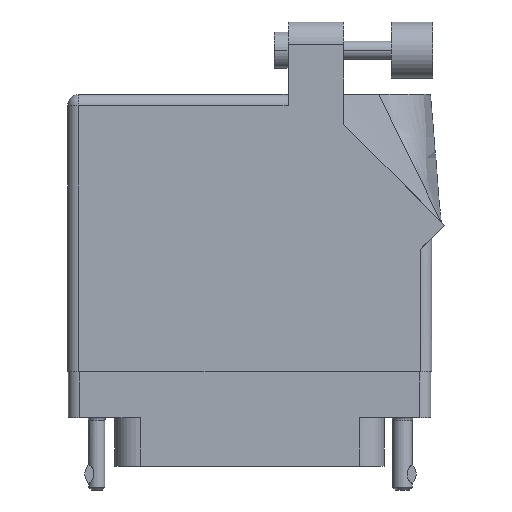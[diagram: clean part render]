
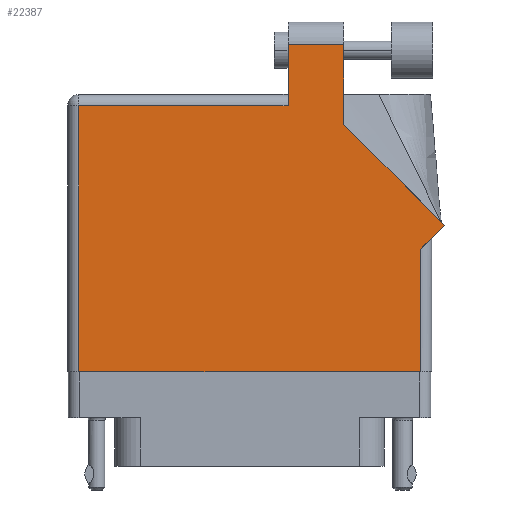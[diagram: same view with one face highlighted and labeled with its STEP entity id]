
A CAD part, front view. The second image highlights one B-rep face of the part: STEP entity #22387.
In plain terms, the highlighted face is planar.
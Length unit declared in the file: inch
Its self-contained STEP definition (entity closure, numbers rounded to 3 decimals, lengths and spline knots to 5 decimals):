
#265 = EDGE_CURVE ( 'NONE', #39136, #20996, #43866, .T. ) ;
#532 = EDGE_CURVE ( 'NONE', #18639, #32042, #30195, .T. ) ;
#1149 = CARTESIAN_POINT ( 'NONE',  ( 0.943, -0.1, 0.455 ) ) ;
#1171 = LINE ( 'NONE', #38625, #28031 ) ;
#1487 = DIRECTION ( 'NONE',  ( 1., 0., 0. ) ) ;
#1673 = CARTESIAN_POINT ( 'NONE',  ( -0.943, -0.1, 0.455 ) ) ;
#2623 = CARTESIAN_POINT ( 'NONE',  ( 0.212, 1.368, 0.455 ) ) ;
#3544 = ORIENTED_EDGE ( 'NONE', *, *, #8520, .T. ) ;
#4183 = ORIENTED_EDGE ( 'NONE', *, *, #13772, .T. ) ;
#4463 = VERTEX_POINT ( 'NONE', #1673 ) ;
#5615 = VECTOR ( 'NONE', #8112, 39.37008 ) ;
#5845 = PLANE ( 'NONE',  #21014 ) ;
#7066 = CARTESIAN_POINT ( 'NONE',  ( 0.943, 0.575, 0.455 ) ) ;
#7652 = VERTEX_POINT ( 'NONE', #2623 ) ;
#7883 = DIRECTION ( 'NONE',  ( -1., 0., 0. ) ) ;
#8112 = DIRECTION ( 'NONE',  ( 0.707, 0.707, 0. ) ) ;
#8467 = EDGE_CURVE ( 'NONE', #43253, #4463, #43627, .T. ) ;
#8520 = EDGE_CURVE ( 'NONE', #4463, #28490, #17906, .T. ) ;
#8932 = ORIENTED_EDGE ( 'NONE', *, *, #25305, .T. ) ;
#8941 = VECTOR ( 'NONE', #26230, 39.37008 ) ;
#9267 = CARTESIAN_POINT ( 'NONE',  ( 0.212, 1.705, 0.455 ) ) ;
#9564 = ORIENTED_EDGE ( 'NONE', *, *, #265, .T. ) ;
#10597 = LINE ( 'NONE', #32821, #8941 ) ;
#10769 = VECTOR ( 'NONE', #27896, 39.37008 ) ;
#13772 = EDGE_CURVE ( 'NONE', #20996, #18639, #31195, .T. ) ;
#14037 = CARTESIAN_POINT ( 'NONE',  ( 0.519, 1.26442, 0.455 ) ) ;
#15099 = CARTESIAN_POINT ( 'NONE',  ( -0.943, -0.1, 0.455 ) ) ;
#16652 = DIRECTION ( 'NONE',  ( -1., 0., 0. ) ) ;
#17893 = LINE ( 'NONE', #20901, #10769 ) ;
#17906 = LINE ( 'NONE', #26004, #32177 ) ;
#18501 = DIRECTION ( 'NONE',  ( 0., -1., 0. ) ) ;
#18639 = VERTEX_POINT ( 'NONE', #24933 ) ;
#20701 = VECTOR ( 'NONE', #18501, 39.37008 ) ;
#20901 = CARTESIAN_POINT ( 'NONE',  ( 0.943, 0.637, 0.455 ) ) ;
#20996 = VERTEX_POINT ( 'NONE', #33366 ) ;
#21014 = AXIS2_PLACEMENT_3D ( 'NONE', #30618, #40550, #16652 ) ;
#21344 = ORIENTED_EDGE ( 'NONE', *, *, #8467, .T. ) ;
#22387 = ADVANCED_FACE ( 'NONE', ( #24769 ), #5845, .F. ) ;
#23096 = CARTESIAN_POINT ( 'NONE',  ( 1.07571, 0.70771, 0.455 ) ) ;
#23632 = VECTOR ( 'NONE', #40493, 39.37008 ) ;
#24769 = FACE_OUTER_BOUND ( 'NONE', #45059, .T. ) ;
#24906 = EDGE_CURVE ( 'NONE', #40046, #39136, #28618, .T. ) ;
#24933 = CARTESIAN_POINT ( 'NONE',  ( 0.519, 1.705, 0.455 ) ) ;
#25305 = EDGE_CURVE ( 'NONE', #7652, #43253, #1171, .T. ) ;
#25799 = VECTOR ( 'NONE', #44161, 39.37008 ) ;
#26004 = CARTESIAN_POINT ( 'NONE',  ( -1.005, -0.1, 0.455 ) ) ;
#26230 = DIRECTION ( 'NONE',  ( 0., -1., 0. ) ) ;
#27896 = DIRECTION ( 'NONE',  ( 0., 1., 0. ) ) ;
#28031 = VECTOR ( 'NONE', #7883, 39.37008 ) ;
#28490 = VERTEX_POINT ( 'NONE', #1149 ) ;
#28618 = LINE ( 'NONE', #35818, #5615 ) ;
#30195 = LINE ( 'NONE', #9267, #25799 ) ;
#30618 = CARTESIAN_POINT ( 'NONE',  ( -1.005, 1.43, 0.455 ) ) ;
#31195 = LINE ( 'NONE', #14037, #33373 ) ;
#31526 = DIRECTION ( 'NONE',  ( 0., 1., 0. ) ) ;
#32042 = VERTEX_POINT ( 'NONE', #44549 ) ;
#32177 = VECTOR ( 'NONE', #1487, 39.37008 ) ;
#32821 = CARTESIAN_POINT ( 'NONE',  ( 0.212, 1.43, 0.455 ) ) ;
#33366 = CARTESIAN_POINT ( 'NONE',  ( 0.519, 1.26442, 0.455 ) ) ;
#33373 = VECTOR ( 'NONE', #31526, 39.37008 ) ;
#33457 = ORIENTED_EDGE ( 'NONE', *, *, #532, .T. ) ;
#35353 = EDGE_CURVE ( 'NONE', #28490, #40046, #17893, .T. ) ;
#35818 = CARTESIAN_POINT ( 'NONE',  ( 1.005, 0.637, 0.455 ) ) ;
#36095 = ORIENTED_EDGE ( 'NONE', *, *, #37046, .T. ) ;
#36755 = ORIENTED_EDGE ( 'NONE', *, *, #35353, .T. ) ;
#37046 = EDGE_CURVE ( 'NONE', #32042, #7652, #10597, .T. ) ;
#38625 = CARTESIAN_POINT ( 'NONE',  ( -1.005, 1.368, 0.455 ) ) ;
#39136 = VERTEX_POINT ( 'NONE', #42745 ) ;
#40046 = VERTEX_POINT ( 'NONE', #7066 ) ;
#40493 = DIRECTION ( 'NONE',  ( -0.707, 0.707, 0. ) ) ;
#40550 = DIRECTION ( 'NONE',  ( 0., 0., -1. ) ) ;
#40602 = CARTESIAN_POINT ( 'NONE',  ( -0.943, 1.368, 0.455 ) ) ;
#42745 = CARTESIAN_POINT ( 'NONE',  ( 1.07571, 0.70771, 0.455 ) ) ;
#43253 = VERTEX_POINT ( 'NONE', #40602 ) ;
#43627 = LINE ( 'NONE', #15099, #20701 ) ;
#43866 = LINE ( 'NONE', #23096, #23632 ) ;
#44161 = DIRECTION ( 'NONE',  ( -1., 0., 0. ) ) ;
#44549 = CARTESIAN_POINT ( 'NONE',  ( 0.212, 1.705, 0.455 ) ) ;
#45059 = EDGE_LOOP ( 'NONE', ( #4183, #33457, #36095, #8932, #21344, #3544, #36755, #45236, #9564 ) ) ;
#45236 = ORIENTED_EDGE ( 'NONE', *, *, #24906, .T. ) ;
